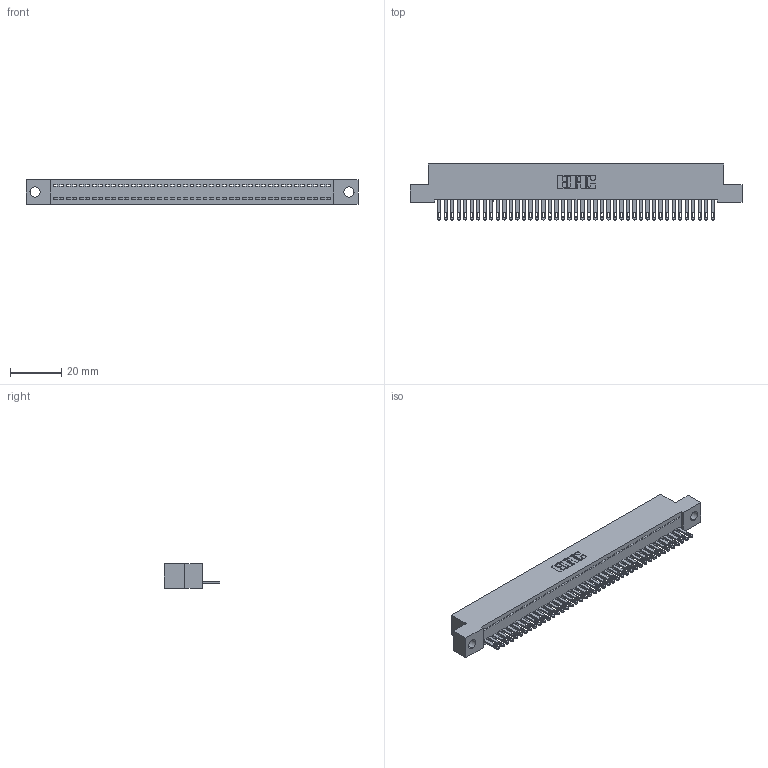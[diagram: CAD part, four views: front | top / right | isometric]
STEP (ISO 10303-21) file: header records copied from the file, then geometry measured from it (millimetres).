
FILE_DESCRIPTION (( 'STEP AP203' ), '1' );
FILE_NAME ('342-043-500-104.STEP', '2019-10-02T18:24:27', ( '' ), ( '' ), 'SwSTEP 2.0', 'SolidWorks 2016', '' );
FILE_SCHEMA (( 'CONFIG_CONTROL_DESIGN' ));
Length unit declared in the file: inch
Products named in the file (3): 342 Part_.156 TH; 345-292-001_345-293-100; 342-043-500-104
Assembly tree (44 placements, depth 2):
  342-043-500-104
    342 Part_.156 TH
    345-292-001_345-293-100  x43
Bounding box: 129.54 x 21.85 x 9.4 mm (x, y, z)
Volume: 11301.3 mm3; surface area: 16517.6 mm2
Topology: 44 solids, 44 shells, 2432 faces, 7523 edges, 5014 vertices
Faces by surface type: plane 1614, cylinder 818
Entity records: 25959 total; most frequent: CARTESIAN_POINT 4483, ORIENTED_EDGE 4462, DIRECTION 3781, EDGE_CURVE 2231, VECTOR 2099, LINE 2099, VERTEX_POINT 1486, AXIS2_PLACEMENT_3D 841
